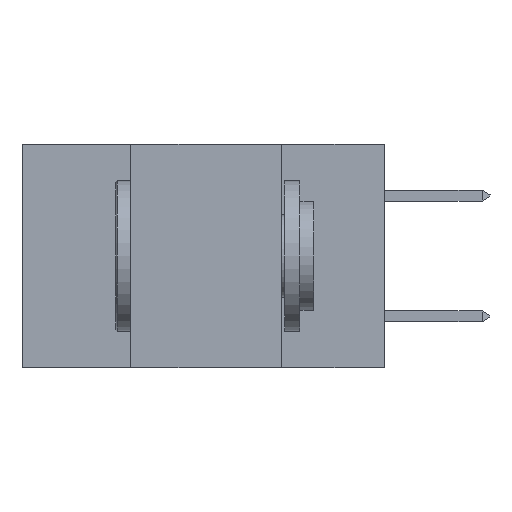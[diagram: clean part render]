
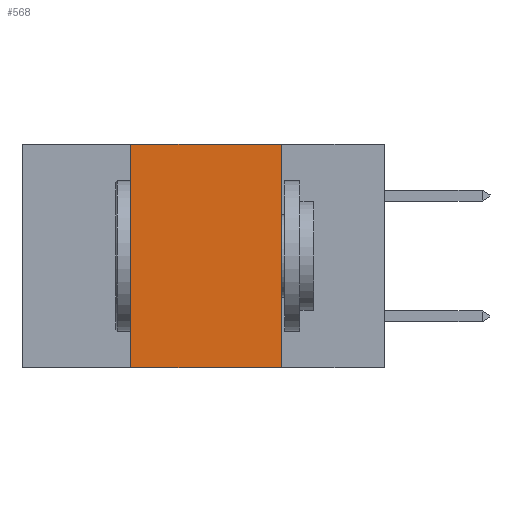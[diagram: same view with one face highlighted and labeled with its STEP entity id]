
A CAD part, left-side view. The second image highlights one B-rep face of the part: STEP entity #568.
In plain terms, the highlighted planar face has unit normal (-1, 0, 0).
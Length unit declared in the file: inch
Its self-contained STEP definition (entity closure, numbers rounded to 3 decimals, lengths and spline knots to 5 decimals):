
#27 = VERTEX_POINT ( 'NONE', #3790 ) ;
#189 = CARTESIAN_POINT ( 'NONE',  ( 0., 0.6, 0. ) ) ;
#568 = ADVANCED_FACE ( 'NONE', ( #8734 ), #2161, .F. ) ;
#727 = EDGE_CURVE ( 'NONE', #9934, #2421, #5550, .T. ) ;
#782 = CARTESIAN_POINT ( 'NONE',  ( 0., 0.17, 0. ) ) ;
#943 = DIRECTION ( 'NONE',  ( 0., -1., 0. ) ) ;
#948 = CARTESIAN_POINT ( 'NONE',  ( 0., 0.42, 0. ) ) ;
#1147 = EDGE_CURVE ( 'NONE', #7160, #9934, #3940, .T. ) ;
#1194 = DIRECTION ( 'NONE',  ( 0., 0., -1. ) ) ;
#1395 = CARTESIAN_POINT ( 'NONE',  ( 0., 0.6, -0.37 ) ) ;
#1520 = VECTOR ( 'NONE', #943, 39.37008 ) ;
#1725 = CARTESIAN_POINT ( 'NONE',  ( 0., 0.42, 0. ) ) ;
#2161 = PLANE ( 'NONE',  #6182 ) ;
#2421 = VERTEX_POINT ( 'NONE', #782 ) ;
#2888 = CARTESIAN_POINT ( 'NONE',  ( 0., 0.17, 0. ) ) ;
#3271 = VECTOR ( 'NONE', #5141, 39.37008 ) ;
#3567 = EDGE_LOOP ( 'NONE', ( #9244, #7843, #9667, #10742 ) ) ;
#3790 = CARTESIAN_POINT ( 'NONE',  ( 0., 0.17, -0.37 ) ) ;
#3940 = LINE ( 'NONE', #1725, #5691 ) ;
#4141 = LINE ( 'NONE', #1395, #5109 ) ;
#4652 = DIRECTION ( 'NONE',  ( 0., 0., 1. ) ) ;
#5109 = VECTOR ( 'NONE', #10404, 39.37008 ) ;
#5141 = DIRECTION ( 'NONE',  ( 0., 0., -1. ) ) ;
#5550 = LINE ( 'NONE', #12184, #1520 ) ;
#5691 = VECTOR ( 'NONE', #4652, 39.37008 ) ;
#6182 = AXIS2_PLACEMENT_3D ( 'NONE', #189, #7271, #1194 ) ;
#7088 = EDGE_CURVE ( 'NONE', #2421, #27, #12898, .T. ) ;
#7160 = VERTEX_POINT ( 'NONE', #9868 ) ;
#7271 = DIRECTION ( 'NONE',  ( 1., 0., 0. ) ) ;
#7843 = ORIENTED_EDGE ( 'NONE', *, *, #727, .F. ) ;
#8734 = FACE_OUTER_BOUND ( 'NONE', #3567, .T. ) ;
#9244 = ORIENTED_EDGE ( 'NONE', *, *, #7088, .F. ) ;
#9667 = ORIENTED_EDGE ( 'NONE', *, *, #1147, .F. ) ;
#9868 = CARTESIAN_POINT ( 'NONE',  ( 0., 0.42, -0.37 ) ) ;
#9934 = VERTEX_POINT ( 'NONE', #948 ) ;
#10404 = DIRECTION ( 'NONE',  ( 0., -1., 0. ) ) ;
#10682 = EDGE_CURVE ( 'NONE', #7160, #27, #4141, .T. ) ;
#10742 = ORIENTED_EDGE ( 'NONE', *, *, #10682, .T. ) ;
#12184 = CARTESIAN_POINT ( 'NONE',  ( 0., 0.6, 0. ) ) ;
#12898 = LINE ( 'NONE', #2888, #3271 ) ;
